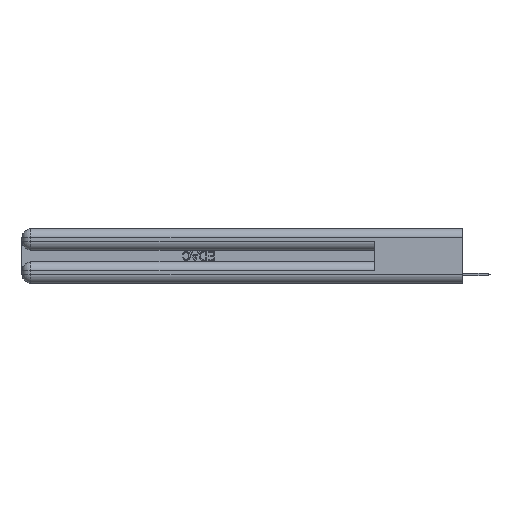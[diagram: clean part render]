
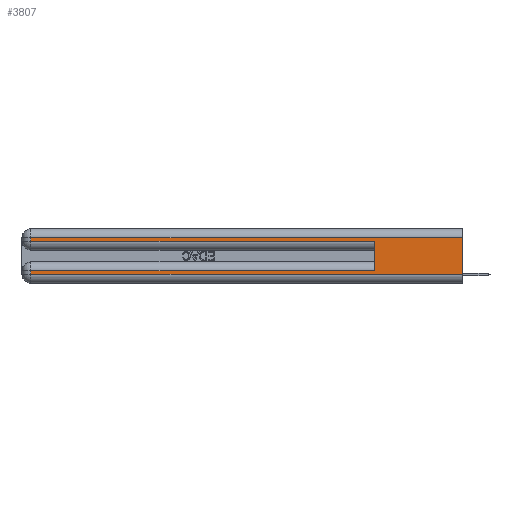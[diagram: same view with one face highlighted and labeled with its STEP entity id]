
A CAD part, left-side view. The second image highlights one B-rep face of the part: STEP entity #3807.
In plain terms, the highlighted planar face has unit normal (-1, 0, 0).
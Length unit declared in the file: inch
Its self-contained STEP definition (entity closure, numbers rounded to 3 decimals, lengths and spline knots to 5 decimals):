
#327 = DIRECTION ( 'NONE',  ( 0., -1., 0. ) ) ;
#403 = LINE ( 'NONE', #6706, #31864 ) ;
#569 = LINE ( 'NONE', #7842, #7955 ) ;
#1620 = VERTEX_POINT ( 'NONE', #30824 ) ;
#2949 = PLANE ( 'NONE',  #21562 ) ;
#3807 = ADVANCED_FACE ( 'NONE', ( #4758 ), #2949, .F. ) ;
#4758 = FACE_OUTER_BOUND ( 'NONE', #15968, .T. ) ;
#4885 = ORIENTED_EDGE ( 'NONE', *, *, #28473, .T. ) ;
#4935 = EDGE_CURVE ( 'NONE', #1620, #30828, #26218, .T. ) ;
#5928 = LINE ( 'NONE', #23684, #10071 ) ;
#6244 = EDGE_CURVE ( 'NONE', #32996, #31794, #403, .T. ) ;
#6706 = CARTESIAN_POINT ( 'NONE',  ( 0., 0.6, 0.145 ) ) ;
#6790 = CARTESIAN_POINT ( 'NONE',  ( 0., 0., 0.06 ) ) ;
#6966 = ORIENTED_EDGE ( 'NONE', *, *, #7506, .T. ) ;
#7390 = EDGE_CURVE ( 'NONE', #12940, #31794, #11117, .T. ) ;
#7506 = EDGE_CURVE ( 'NONE', #19453, #15170, #569, .T. ) ;
#7607 = EDGE_CURVE ( 'NONE', #11019, #1620, #26045, .T. ) ;
#7814 = DIRECTION ( 'NONE',  ( 0., 1., 0. ) ) ;
#7842 = CARTESIAN_POINT ( 'NONE',  ( 0., 0., 0.31 ) ) ;
#7955 = VECTOR ( 'NONE', #29027, 39.37008 ) ;
#8574 = ORIENTED_EDGE ( 'NONE', *, *, #7390, .T. ) ;
#9138 = CARTESIAN_POINT ( 'NONE',  ( 0., 2.94, 0.37 ) ) ;
#9693 = EDGE_CURVE ( 'NONE', #19453, #30828, #28383, .T. ) ;
#10071 = VECTOR ( 'NONE', #7814, 39.37008 ) ;
#10221 = EDGE_CURVE ( 'NONE', #15170, #12940, #24206, .T. ) ;
#10267 = ORIENTED_EDGE ( 'NONE', *, *, #10221, .T. ) ;
#11019 = VERTEX_POINT ( 'NONE', #18931 ) ;
#11117 = LINE ( 'NONE', #13238, #24367 ) ;
#12940 = VERTEX_POINT ( 'NONE', #29495 ) ;
#13238 = CARTESIAN_POINT ( 'NONE',  ( 0., 0., 0.285 ) ) ;
#14453 = DIRECTION ( 'NONE',  ( 0., 0., -1. ) ) ;
#15170 = VERTEX_POINT ( 'NONE', #32309 ) ;
#15968 = EDGE_LOOP ( 'NONE', ( #31587, #6966, #10267, #8574, #30793, #4885, #28366, #19308 ) ) ;
#18133 = VECTOR ( 'NONE', #34168, 39.37008 ) ;
#18931 = CARTESIAN_POINT ( 'NONE',  ( 0., 2.94, 0.085 ) ) ;
#19252 = VECTOR ( 'NONE', #27392, 39.37008 ) ;
#19308 = ORIENTED_EDGE ( 'NONE', *, *, #4935, .T. ) ;
#19453 = VERTEX_POINT ( 'NONE', #33637 ) ;
#20236 = DIRECTION ( 'NONE',  ( 0., 0., 1. ) ) ;
#21562 = AXIS2_PLACEMENT_3D ( 'NONE', #21804, #31986, #31868 ) ;
#21804 = CARTESIAN_POINT ( 'NONE',  ( 0., 0., 0.37 ) ) ;
#23402 = CARTESIAN_POINT ( 'NONE',  ( 0., 2.94, 0.37 ) ) ;
#23684 = CARTESIAN_POINT ( 'NONE',  ( 0., 0., 0.085 ) ) ;
#23809 = CARTESIAN_POINT ( 'NONE',  ( 0., 0., 0.06 ) ) ;
#24206 = LINE ( 'NONE', #9138, #33749 ) ;
#24367 = VECTOR ( 'NONE', #327, 39.37008 ) ;
#25629 = CARTESIAN_POINT ( 'NONE',  ( 0., 0.6, 0.085 ) ) ;
#26045 = LINE ( 'NONE', #23402, #18133 ) ;
#26218 = LINE ( 'NONE', #6790, #32397 ) ;
#27392 = DIRECTION ( 'NONE',  ( 0., 0., -1. ) ) ;
#28366 = ORIENTED_EDGE ( 'NONE', *, *, #7607, .T. ) ;
#28383 = LINE ( 'NONE', #32219, #19252 ) ;
#28473 = EDGE_CURVE ( 'NONE', #32996, #11019, #5928, .T. ) ;
#28704 = CARTESIAN_POINT ( 'NONE',  ( 0., 0.6, 0.285 ) ) ;
#29027 = DIRECTION ( 'NONE',  ( 0., 1., 0. ) ) ;
#29495 = CARTESIAN_POINT ( 'NONE',  ( 0., 2.94, 0.285 ) ) ;
#30178 = DIRECTION ( 'NONE',  ( 0., -1., 0. ) ) ;
#30793 = ORIENTED_EDGE ( 'NONE', *, *, #6244, .F. ) ;
#30824 = CARTESIAN_POINT ( 'NONE',  ( 0., 2.94, 0.06 ) ) ;
#30828 = VERTEX_POINT ( 'NONE', #23809 ) ;
#31587 = ORIENTED_EDGE ( 'NONE', *, *, #9693, .F. ) ;
#31794 = VERTEX_POINT ( 'NONE', #28704 ) ;
#31864 = VECTOR ( 'NONE', #20236, 39.37008 ) ;
#31868 = DIRECTION ( 'NONE',  ( 0., 0., -1. ) ) ;
#31986 = DIRECTION ( 'NONE',  ( 1., 0., 0. ) ) ;
#32219 = CARTESIAN_POINT ( 'NONE',  ( 0., 0., 0.37 ) ) ;
#32309 = CARTESIAN_POINT ( 'NONE',  ( 0., 2.94, 0.31 ) ) ;
#32397 = VECTOR ( 'NONE', #30178, 39.37008 ) ;
#32996 = VERTEX_POINT ( 'NONE', #25629 ) ;
#33637 = CARTESIAN_POINT ( 'NONE',  ( 0., 0., 0.31 ) ) ;
#33749 = VECTOR ( 'NONE', #14453, 39.37008 ) ;
#34168 = DIRECTION ( 'NONE',  ( 0., 0., -1. ) ) ;
